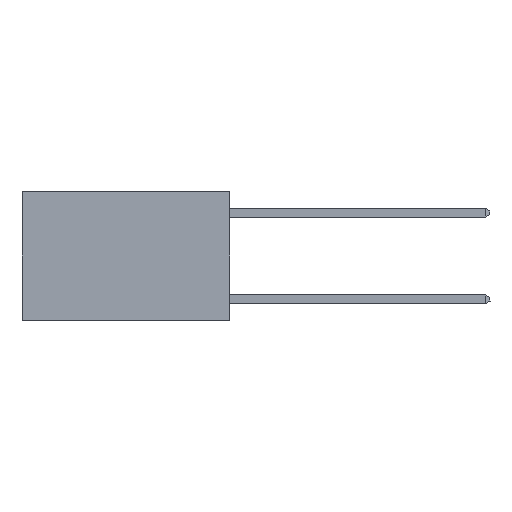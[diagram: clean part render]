
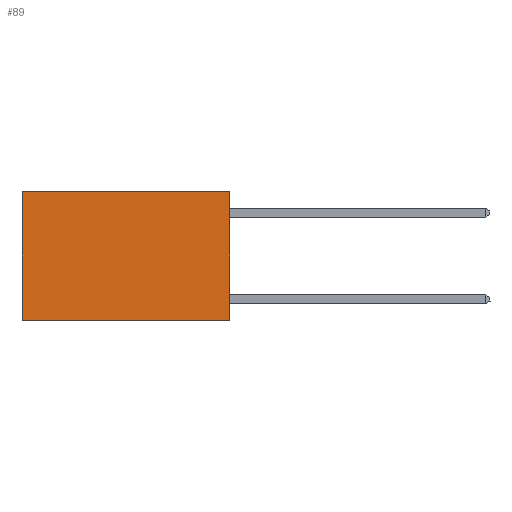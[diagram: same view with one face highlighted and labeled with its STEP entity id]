
A CAD part, left-side view. The second image highlights one B-rep face of the part: STEP entity #89.
In plain terms, the highlighted planar face has unit normal (-1, 0, 0).
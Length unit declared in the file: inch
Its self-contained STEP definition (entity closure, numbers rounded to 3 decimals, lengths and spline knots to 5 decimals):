
#89 = ADVANCED_FACE ( 'NONE', ( #26394 ), #5957, .F. ) ;
#877 = EDGE_CURVE ( 'NONE', #1920, #4087, #15403, .T. ) ;
#1137 = LINE ( 'NONE', #18306, #17118 ) ;
#1147 = EDGE_CURVE ( 'NONE', #27264, #17817, #1137, .T. ) ;
#1590 = DIRECTION ( 'NONE',  ( 0., 0., -1. ) ) ;
#1920 = VERTEX_POINT ( 'NONE', #6284 ) ;
#3220 = EDGE_CURVE ( 'NONE', #17817, #4087, #19769, .T. ) ;
#4087 = VERTEX_POINT ( 'NONE', #6040 ) ;
#4853 = ORIENTED_EDGE ( 'NONE', *, *, #17161, .F. ) ;
#4919 = CARTESIAN_POINT ( 'NONE',  ( 0.2625, 0.6, 0. ) ) ;
#5957 = PLANE ( 'NONE',  #6277 ) ;
#6040 = CARTESIAN_POINT ( 'NONE',  ( 0.2625, 0.6, -0.37 ) ) ;
#6277 = AXIS2_PLACEMENT_3D ( 'NONE', #19166, #21374, #1590 ) ;
#6284 = CARTESIAN_POINT ( 'NONE',  ( 0.2625, 0., -0.37 ) ) ;
#6721 = CARTESIAN_POINT ( 'NONE',  ( 0.2625, 0., 0. ) ) ;
#7743 = EDGE_LOOP ( 'NONE', ( #19026, #16038, #4853, #16206 ) ) ;
#8171 = VECTOR ( 'NONE', #23791, 39.37008 ) ;
#11083 = DIRECTION ( 'NONE',  ( 0., 0., -1. ) ) ;
#15068 = VECTOR ( 'NONE', #11083, 39.37008 ) ;
#15403 = LINE ( 'NONE', #21911, #24971 ) ;
#16038 = ORIENTED_EDGE ( 'NONE', *, *, #877, .F. ) ;
#16206 = ORIENTED_EDGE ( 'NONE', *, *, #1147, .T. ) ;
#16392 = DIRECTION ( 'NONE',  ( 0., 1., 0. ) ) ;
#17118 = VECTOR ( 'NONE', #16392, 39.37008 ) ;
#17161 = EDGE_CURVE ( 'NONE', #27264, #1920, #24623, .T. ) ;
#17817 = VERTEX_POINT ( 'NONE', #4919 ) ;
#18306 = CARTESIAN_POINT ( 'NONE',  ( 0.2625, 0., 0. ) ) ;
#19026 = ORIENTED_EDGE ( 'NONE', *, *, #3220, .T. ) ;
#19166 = CARTESIAN_POINT ( 'NONE',  ( 0.2625, 0., 0. ) ) ;
#19769 = LINE ( 'NONE', #26196, #8171 ) ;
#21374 = DIRECTION ( 'NONE',  ( 1., 0., 0. ) ) ;
#21911 = CARTESIAN_POINT ( 'NONE',  ( 0.2625, 0., -0.37 ) ) ;
#22856 = CARTESIAN_POINT ( 'NONE',  ( 0.2625, 0., 0. ) ) ;
#23791 = DIRECTION ( 'NONE',  ( 0., 0., -1. ) ) ;
#23911 = DIRECTION ( 'NONE',  ( 0., 1., 0. ) ) ;
#24623 = LINE ( 'NONE', #6721, #15068 ) ;
#24971 = VECTOR ( 'NONE', #23911, 39.37008 ) ;
#26196 = CARTESIAN_POINT ( 'NONE',  ( 0.2625, 0.6, 0. ) ) ;
#26394 = FACE_OUTER_BOUND ( 'NONE', #7743, .T. ) ;
#27264 = VERTEX_POINT ( 'NONE', #22856 ) ;
